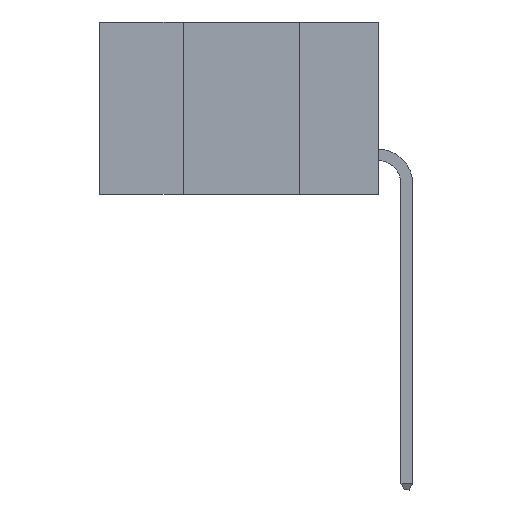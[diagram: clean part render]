
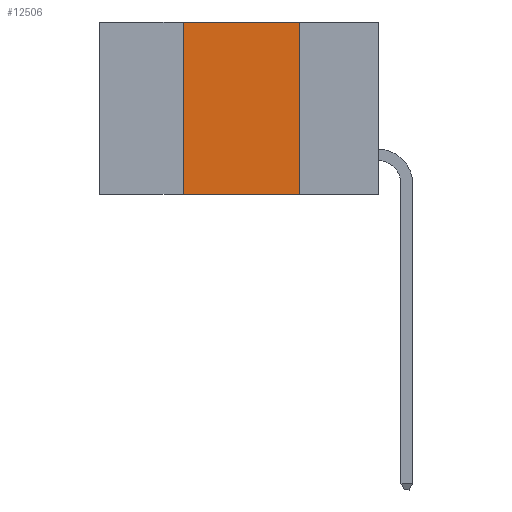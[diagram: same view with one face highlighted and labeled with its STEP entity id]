
A CAD part, left-side view. The second image highlights one B-rep face of the part: STEP entity #12506.
In plain terms, the highlighted planar face has unit normal (-1, 0, 0).
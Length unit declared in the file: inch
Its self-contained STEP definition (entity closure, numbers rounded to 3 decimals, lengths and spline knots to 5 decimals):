
#53 = DIRECTION ( 'NONE',  ( 0., -1., 0. ) ) ;
#704 = DIRECTION ( 'NONE',  ( 1., 0., 0. ) ) ;
#1628 = LINE ( 'NONE', #6101, #12880 ) ;
#1698 = DIRECTION ( 'NONE',  ( 0., -1., 0. ) ) ;
#2241 = VECTOR ( 'NONE', #1698, 39.37008 ) ;
#2511 = CARTESIAN_POINT ( 'NONE',  ( 0., 0.6, -0.37 ) ) ;
#3362 = EDGE_CURVE ( 'NONE', #11151, #11627, #7672, .T. ) ;
#3824 = VECTOR ( 'NONE', #53, 39.37008 ) ;
#4409 = CARTESIAN_POINT ( 'NONE',  ( 0., 0.42, 0. ) ) ;
#4734 = VECTOR ( 'NONE', #6686, 39.37008 ) ;
#4958 = CARTESIAN_POINT ( 'NONE',  ( 0., 0.42, -0.37 ) ) ;
#5212 = ORIENTED_EDGE ( 'NONE', *, *, #7017, .F. ) ;
#5869 = FACE_OUTER_BOUND ( 'NONE', #17257, .T. ) ;
#6101 = CARTESIAN_POINT ( 'NONE',  ( 0., 0.42, 0. ) ) ;
#6415 = VERTEX_POINT ( 'NONE', #4409 ) ;
#6569 = CARTESIAN_POINT ( 'NONE',  ( 0., 0.17, 0. ) ) ;
#6686 = DIRECTION ( 'NONE',  ( 0., 0., -1. ) ) ;
#6953 = AXIS2_PLACEMENT_3D ( 'NONE', #17924, #704, #10987 ) ;
#7017 = EDGE_CURVE ( 'NONE', #15049, #11627, #8609, .T. ) ;
#7672 = LINE ( 'NONE', #2511, #3824 ) ;
#8003 = PLANE ( 'NONE',  #6953 ) ;
#8609 = LINE ( 'NONE', #6569, #4734 ) ;
#8719 = EDGE_CURVE ( 'NONE', #11151, #6415, #1628, .T. ) ;
#10379 = CARTESIAN_POINT ( 'NONE',  ( 0., 0.17, -0.37 ) ) ;
#10526 = CARTESIAN_POINT ( 'NONE',  ( 0., 0.6, 0. ) ) ;
#10987 = DIRECTION ( 'NONE',  ( 0., 0., -1. ) ) ;
#11001 = EDGE_CURVE ( 'NONE', #6415, #15049, #13466, .T. ) ;
#11151 = VERTEX_POINT ( 'NONE', #4958 ) ;
#11627 = VERTEX_POINT ( 'NONE', #10379 ) ;
#12506 = ADVANCED_FACE ( 'NONE', ( #5869 ), #8003, .F. ) ;
#12880 = VECTOR ( 'NONE', #17434, 39.37008 ) ;
#13172 = CARTESIAN_POINT ( 'NONE',  ( 0., 0.17, 0. ) ) ;
#13466 = LINE ( 'NONE', #10526, #2241 ) ;
#13863 = ORIENTED_EDGE ( 'NONE', *, *, #8719, .F. ) ;
#14301 = ORIENTED_EDGE ( 'NONE', *, *, #3362, .T. ) ;
#15049 = VERTEX_POINT ( 'NONE', #13172 ) ;
#17257 = EDGE_LOOP ( 'NONE', ( #5212, #17509, #13863, #14301 ) ) ;
#17434 = DIRECTION ( 'NONE',  ( 0., 0., 1. ) ) ;
#17509 = ORIENTED_EDGE ( 'NONE', *, *, #11001, .F. ) ;
#17924 = CARTESIAN_POINT ( 'NONE',  ( 0., 0.6, 0. ) ) ;
